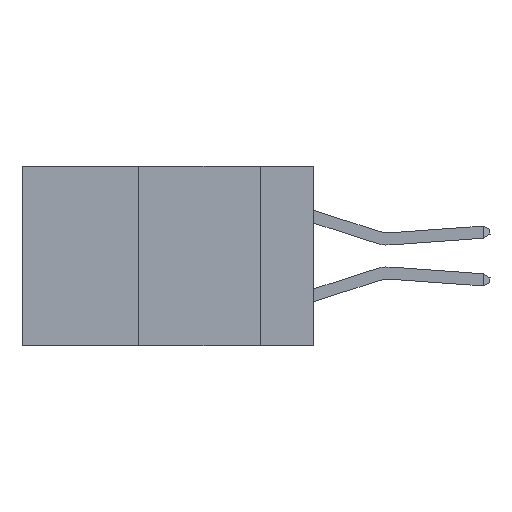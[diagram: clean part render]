
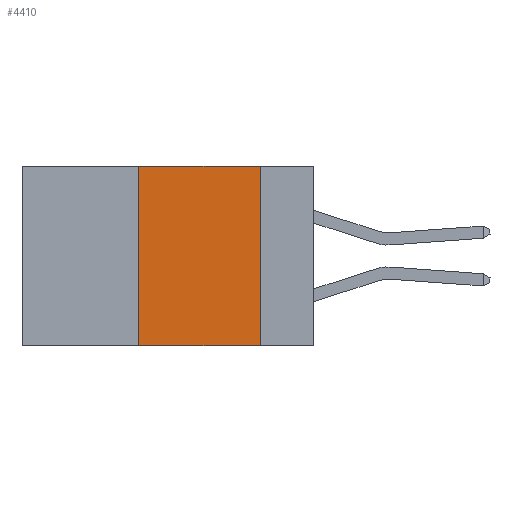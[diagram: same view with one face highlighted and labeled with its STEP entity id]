
A CAD part, left-side view. The second image highlights one B-rep face of the part: STEP entity #4410.
In plain terms, the highlighted planar face has unit normal (-1, 0, 0).
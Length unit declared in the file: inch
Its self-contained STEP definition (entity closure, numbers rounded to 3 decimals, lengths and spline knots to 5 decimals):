
#2175 = DIRECTION ( 'NONE',  ( 0., 0., -1. ) ) ;
#3436 = EDGE_CURVE ( 'NONE', #15019, #8134, #19811, .T. ) ;
#4410 = ADVANCED_FACE ( 'NONE', ( #14503 ), #19114, .F. ) ;
#5575 = DIRECTION ( 'NONE',  ( 0., 0., -1. ) ) ;
#5835 = DIRECTION ( 'NONE',  ( 0., 0., 1. ) ) ;
#6356 = DIRECTION ( 'NONE',  ( 0., -1., 0. ) ) ;
#6759 = AXIS2_PLACEMENT_3D ( 'NONE', #10514, #10668, #2175 ) ;
#7344 = EDGE_CURVE ( 'NONE', #8134, #14733, #19664, .T. ) ;
#7749 = ORIENTED_EDGE ( 'NONE', *, *, #9348, .T. ) ;
#8134 = VERTEX_POINT ( 'NONE', #21545 ) ;
#9149 = EDGE_LOOP ( 'NONE', ( #10666, #12565, #9180, #7749 ) ) ;
#9180 = ORIENTED_EDGE ( 'NONE', *, *, #3436, .F. ) ;
#9348 = EDGE_CURVE ( 'NONE', #15019, #21832, #16131, .T. ) ;
#9942 = EDGE_CURVE ( 'NONE', #14733, #21832, #14565, .T. ) ;
#10102 = VECTOR ( 'NONE', #16778, 39.37008 ) ;
#10502 = CARTESIAN_POINT ( 'NONE',  ( 0., 0.36, -0.37 ) ) ;
#10514 = CARTESIAN_POINT ( 'NONE',  ( 0., 0.6, 0. ) ) ;
#10666 = ORIENTED_EDGE ( 'NONE', *, *, #9942, .F. ) ;
#10668 = DIRECTION ( 'NONE',  ( 1., 0., 0. ) ) ;
#12131 = VECTOR ( 'NONE', #6356, 39.37008 ) ;
#12561 = CARTESIAN_POINT ( 'NONE',  ( 0., 0.36, 0. ) ) ;
#12565 = ORIENTED_EDGE ( 'NONE', *, *, #7344, .F. ) ;
#14198 = CARTESIAN_POINT ( 'NONE',  ( 0., 0.11, 0. ) ) ;
#14339 = CARTESIAN_POINT ( 'NONE',  ( 0., 0.11, -0.37 ) ) ;
#14503 = FACE_OUTER_BOUND ( 'NONE', #9149, .T. ) ;
#14565 = LINE ( 'NONE', #14198, #18522 ) ;
#14733 = VERTEX_POINT ( 'NONE', #19433 ) ;
#15019 = VERTEX_POINT ( 'NONE', #10502 ) ;
#15277 = VECTOR ( 'NONE', #5835, 39.37008 ) ;
#16131 = LINE ( 'NONE', #16421, #12131 ) ;
#16421 = CARTESIAN_POINT ( 'NONE',  ( 0., 0.6, -0.37 ) ) ;
#16778 = DIRECTION ( 'NONE',  ( 0., -1., 0. ) ) ;
#18275 = CARTESIAN_POINT ( 'NONE',  ( 0., 0.6, 0. ) ) ;
#18522 = VECTOR ( 'NONE', #5575, 39.37008 ) ;
#19114 = PLANE ( 'NONE',  #6759 ) ;
#19433 = CARTESIAN_POINT ( 'NONE',  ( 0., 0.11, 0. ) ) ;
#19664 = LINE ( 'NONE', #18275, #10102 ) ;
#19811 = LINE ( 'NONE', #12561, #15277 ) ;
#21545 = CARTESIAN_POINT ( 'NONE',  ( 0., 0.36, 0. ) ) ;
#21832 = VERTEX_POINT ( 'NONE', #14339 ) ;
